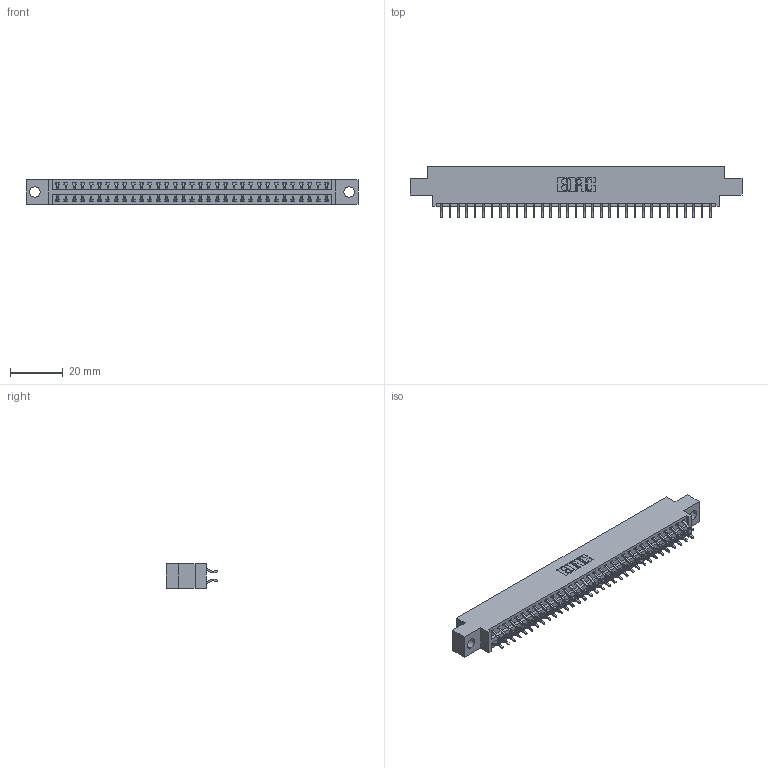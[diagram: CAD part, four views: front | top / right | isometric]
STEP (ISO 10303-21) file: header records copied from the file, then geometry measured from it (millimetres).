
FILE_DESCRIPTION (( 'STEP AP203' ), '1' );
FILE_NAME ('346-066-556-804.STEP', '2022-05-24T17:49:35', ( '' ), ( '' ), 'SwSTEP 2.0', 'SolidWorks 2020', '' );
FILE_SCHEMA (( 'CONFIG_CONTROL_DESIGN' ));
Length unit declared in the file: inch
Products named in the file (3): 346-066-556-804; 346 Part_0.170 Offset - 0.156 Dia-TH; 345-292-001_556 Tail
Assembly tree (67 placements, depth 2):
  346-066-556-804
    346 Part_0.170 Offset - 0.156 Dia-TH
    345-292-001_556 Tail  x66
Bounding box: 125.35 x 19.57 x 9.4 mm (x, y, z)
Volume: 11890 mm3; surface area: 16168.4 mm2
Topology: 67 solids, 67 shells, 3968 faces, 11795 edges, 7774 vertices
Faces by surface type: plane 2668, cylinder 1300
Entity records: 23519 total; most frequent: CARTESIAN_POINT 3910, ORIENTED_EDGE 3830, DIRECTION 3483, EDGE_CURVE 1915, LINE 1643, VECTOR 1643, VERTEX_POINT 1274, AXIS2_PLACEMENT_3D 920
